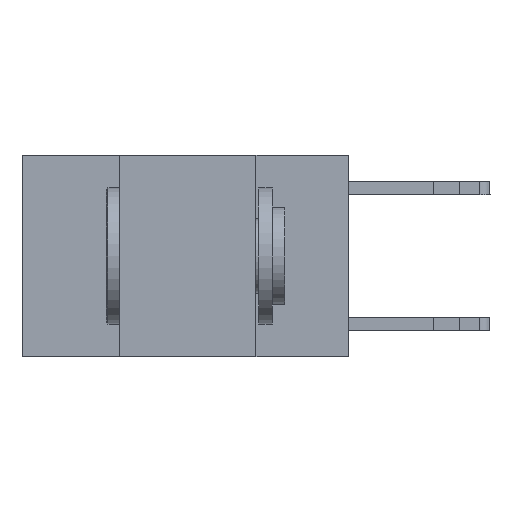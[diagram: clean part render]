
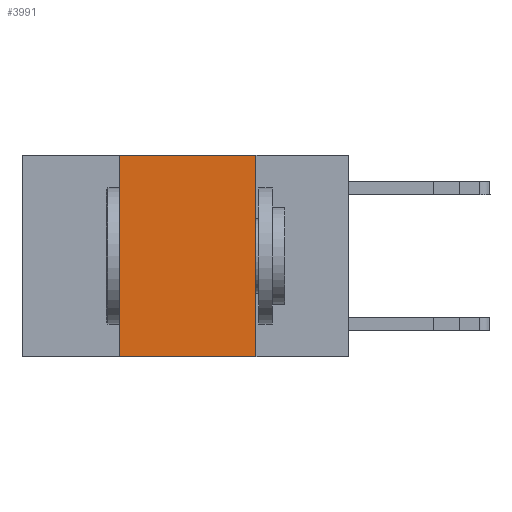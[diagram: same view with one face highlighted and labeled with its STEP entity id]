
A CAD part, left-side view. The second image highlights one B-rep face of the part: STEP entity #3991.
In plain terms, the highlighted planar face has unit normal (-1, 0, 0).
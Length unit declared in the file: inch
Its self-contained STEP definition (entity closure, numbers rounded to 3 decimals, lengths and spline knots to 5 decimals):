
#1066 = LINE ( 'NONE', #11278, #9872 ) ;
#1448 = DIRECTION ( 'NONE',  ( 1., 0., 0. ) ) ;
#1828 = ORIENTED_EDGE ( 'NONE', *, *, #8337, .T. ) ;
#1873 = CARTESIAN_POINT ( 'NONE',  ( 0., 0.42, -0.37 ) ) ;
#2034 = LINE ( 'NONE', #11426, #10464 ) ;
#2207 = CARTESIAN_POINT ( 'NONE',  ( 0., 0.6, 0. ) ) ;
#3336 = DIRECTION ( 'NONE',  ( 0., -1., 0. ) ) ;
#3991 = ADVANCED_FACE ( 'NONE', ( #6571 ), #13435, .F. ) ;
#4329 = CARTESIAN_POINT ( 'NONE',  ( 0., 0.6, -0.37 ) ) ;
#4549 = VERTEX_POINT ( 'NONE', #12146 ) ;
#5840 = EDGE_CURVE ( 'NONE', #12769, #4549, #13802, .T. ) ;
#5871 = DIRECTION ( 'NONE',  ( 0., 0., 1. ) ) ;
#6196 = VERTEX_POINT ( 'NONE', #1873 ) ;
#6427 = VERTEX_POINT ( 'NONE', #10442 ) ;
#6571 = FACE_OUTER_BOUND ( 'NONE', #7345, .T. ) ;
#7345 = EDGE_LOOP ( 'NONE', ( #9930, #10258, #13104, #1828 ) ) ;
#8337 = EDGE_CURVE ( 'NONE', #6196, #6427, #10040, .T. ) ;
#8482 = CARTESIAN_POINT ( 'NONE',  ( 0., 0.42, 0. ) ) ;
#8561 = EDGE_CURVE ( 'NONE', #6196, #12769, #1066, .T. ) ;
#8759 = DIRECTION ( 'NONE',  ( 0., -1., 0. ) ) ;
#9185 = DIRECTION ( 'NONE',  ( 0., 0., -1. ) ) ;
#9715 = VECTOR ( 'NONE', #8759, 39.37008 ) ;
#9872 = VECTOR ( 'NONE', #5871, 39.37008 ) ;
#9930 = ORIENTED_EDGE ( 'NONE', *, *, #12008, .F. ) ;
#10040 = LINE ( 'NONE', #4329, #9715 ) ;
#10258 = ORIENTED_EDGE ( 'NONE', *, *, #5840, .F. ) ;
#10442 = CARTESIAN_POINT ( 'NONE',  ( 0., 0.17, -0.37 ) ) ;
#10464 = VECTOR ( 'NONE', #12493, 39.37008 ) ;
#11278 = CARTESIAN_POINT ( 'NONE',  ( 0., 0.42, 0. ) ) ;
#11426 = CARTESIAN_POINT ( 'NONE',  ( 0., 0.17, 0. ) ) ;
#12008 = EDGE_CURVE ( 'NONE', #4549, #6427, #2034, .T. ) ;
#12146 = CARTESIAN_POINT ( 'NONE',  ( 0., 0.17, 0. ) ) ;
#12350 = CARTESIAN_POINT ( 'NONE',  ( 0., 0.6, 0. ) ) ;
#12493 = DIRECTION ( 'NONE',  ( 0., 0., -1. ) ) ;
#12769 = VERTEX_POINT ( 'NONE', #8482 ) ;
#13104 = ORIENTED_EDGE ( 'NONE', *, *, #8561, .F. ) ;
#13118 = VECTOR ( 'NONE', #3336, 39.37008 ) ;
#13296 = AXIS2_PLACEMENT_3D ( 'NONE', #12350, #1448, #9185 ) ;
#13435 = PLANE ( 'NONE',  #13296 ) ;
#13802 = LINE ( 'NONE', #2207, #13118 ) ;
